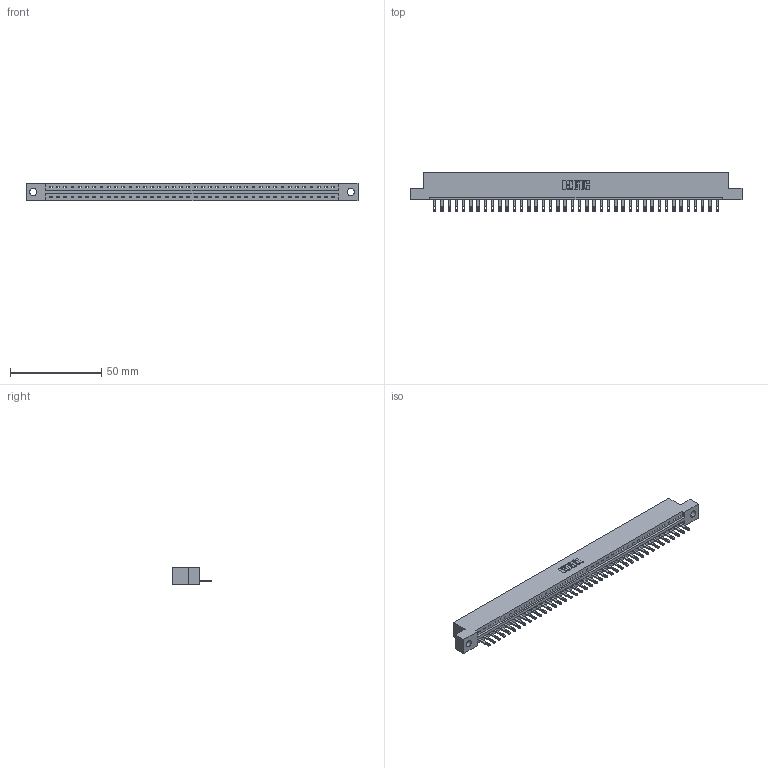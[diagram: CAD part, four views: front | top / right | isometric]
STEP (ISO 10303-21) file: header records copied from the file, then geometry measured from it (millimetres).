
FILE_DESCRIPTION (( 'STEP AP203' ), '1' );
FILE_NAME ('887-040-500-104.STEP', '2020-09-20T23:16:38', ( '' ), ( '' ), 'SwSTEP 2.0', 'SolidWorks 2020', '' );
FILE_SCHEMA (( 'CONFIG_CONTROL_DESIGN' ));
Length unit declared in the file: inch
Products named in the file (3): 345-292-001_345-293-100; 837 Part_Flush Mounting Lugs - 0.156 Dia-TH; 887-040-500-104
Assembly tree (41 placements, depth 2):
  887-040-500-104
    837 Part_Flush Mounting Lugs - 0.156 Dia-TH
    345-292-001_345-293-100  x40
Bounding box: 181.51 x 21.85 x 9.4 mm (x, y, z)
Volume: 18776.6 mm3; surface area: 19280.4 mm2
Topology: 41 solids, 41 shells, 2434 faces, 7511 edges, 5006 vertices
Faces by surface type: plane 1670, cylinder 764
Entity records: 29925 total; most frequent: CARTESIAN_POINT 5218, ORIENTED_EDGE 5194, DIRECTION 4397, EDGE_CURVE 2597, VECTOR 2465, LINE 2465, VERTEX_POINT 1730, AXIS2_PLACEMENT_3D 966
